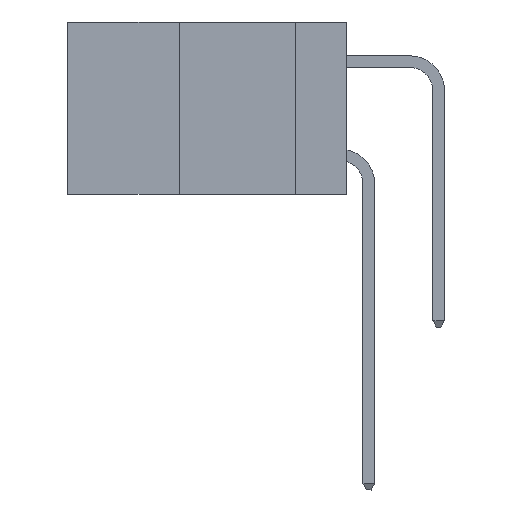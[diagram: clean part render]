
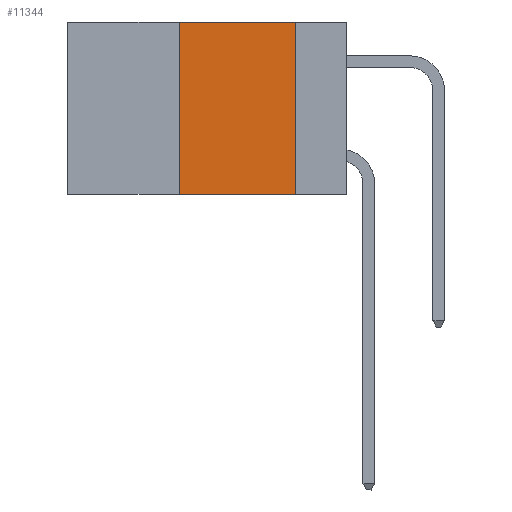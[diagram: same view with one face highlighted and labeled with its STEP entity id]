
A CAD part, left-side view. The second image highlights one B-rep face of the part: STEP entity #11344.
In plain terms, the highlighted planar face has unit normal (-1, 0, 0).
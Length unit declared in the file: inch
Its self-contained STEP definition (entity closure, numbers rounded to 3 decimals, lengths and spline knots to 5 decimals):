
#99 = FACE_OUTER_BOUND ( 'NONE', #14349, .T. ) ;
#145 = LINE ( 'NONE', #4950, #6816 ) ;
#753 = CARTESIAN_POINT ( 'NONE',  ( 0., 0.36, 0. ) ) ;
#2545 = CARTESIAN_POINT ( 'NONE',  ( 0., 0.6, 0. ) ) ;
#2719 = AXIS2_PLACEMENT_3D ( 'NONE', #8339, #13335, #7143 ) ;
#2741 = VECTOR ( 'NONE', #13044, 39.37008 ) ;
#2968 = VERTEX_POINT ( 'NONE', #4629 ) ;
#3200 = VERTEX_POINT ( 'NONE', #753 ) ;
#3495 = DIRECTION ( 'NONE',  ( 0., -1., 0. ) ) ;
#3523 = CARTESIAN_POINT ( 'NONE',  ( 0., 0.36, 0. ) ) ;
#3595 = LINE ( 'NONE', #3523, #2741 ) ;
#3802 = DIRECTION ( 'NONE',  ( 0., -1., 0. ) ) ;
#3814 = EDGE_CURVE ( 'NONE', #10018, #7453, #4750, .T. ) ;
#4130 = ORIENTED_EDGE ( 'NONE', *, *, #3814, .T. ) ;
#4629 = CARTESIAN_POINT ( 'NONE',  ( 0., 0.11, 0. ) ) ;
#4674 = PLANE ( 'NONE',  #2719 ) ;
#4750 = LINE ( 'NONE', #11761, #10127 ) ;
#4950 = CARTESIAN_POINT ( 'NONE',  ( 0., 0.11, 0. ) ) ;
#6351 = ORIENTED_EDGE ( 'NONE', *, *, #13962, .F. ) ;
#6491 = VECTOR ( 'NONE', #3802, 39.37008 ) ;
#6816 = VECTOR ( 'NONE', #7182, 39.37008 ) ;
#7143 = DIRECTION ( 'NONE',  ( 0., 0., -1. ) ) ;
#7182 = DIRECTION ( 'NONE',  ( 0., 0., -1. ) ) ;
#7213 = ORIENTED_EDGE ( 'NONE', *, *, #14723, .F. ) ;
#7453 = VERTEX_POINT ( 'NONE', #12511 ) ;
#8339 = CARTESIAN_POINT ( 'NONE',  ( 0., 0.6, 0. ) ) ;
#9849 = LINE ( 'NONE', #2545, #6491 ) ;
#9867 = ORIENTED_EDGE ( 'NONE', *, *, #9957, .F. ) ;
#9957 = EDGE_CURVE ( 'NONE', #3200, #2968, #9849, .T. ) ;
#10018 = VERTEX_POINT ( 'NONE', #11354 ) ;
#10127 = VECTOR ( 'NONE', #3495, 39.37008 ) ;
#11344 = ADVANCED_FACE ( 'NONE', ( #99 ), #4674, .F. ) ;
#11354 = CARTESIAN_POINT ( 'NONE',  ( 0., 0.36, -0.37 ) ) ;
#11761 = CARTESIAN_POINT ( 'NONE',  ( 0., 0.6, -0.37 ) ) ;
#12511 = CARTESIAN_POINT ( 'NONE',  ( 0., 0.11, -0.37 ) ) ;
#13044 = DIRECTION ( 'NONE',  ( 0., 0., 1. ) ) ;
#13335 = DIRECTION ( 'NONE',  ( 1., 0., 0. ) ) ;
#13962 = EDGE_CURVE ( 'NONE', #10018, #3200, #3595, .T. ) ;
#14349 = EDGE_LOOP ( 'NONE', ( #7213, #9867, #6351, #4130 ) ) ;
#14723 = EDGE_CURVE ( 'NONE', #2968, #7453, #145, .T. ) ;
